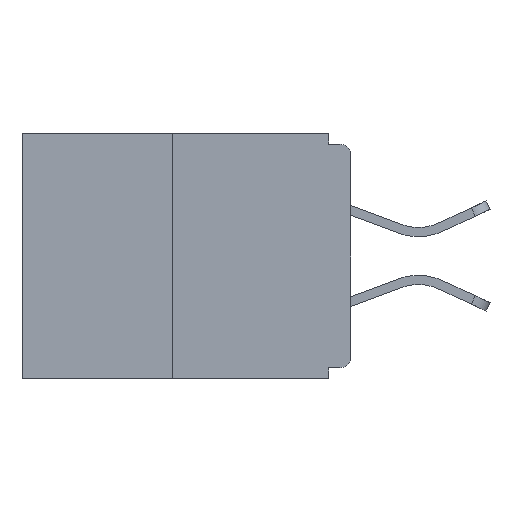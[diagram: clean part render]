
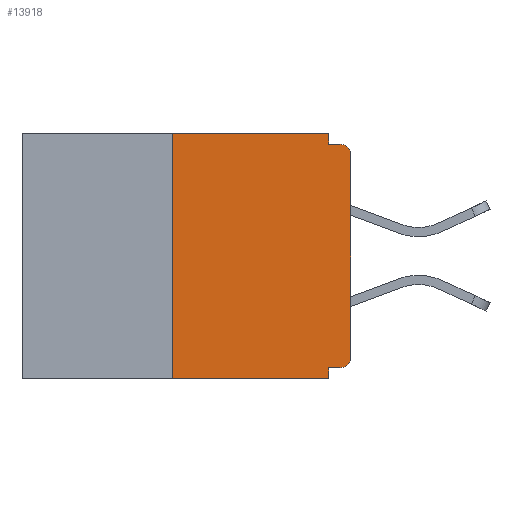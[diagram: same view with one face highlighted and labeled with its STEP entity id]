
A CAD part, left-side view. The second image highlights one B-rep face of the part: STEP entity #13918.
In plain terms, the highlighted planar face has unit normal (-1, 0, 0).
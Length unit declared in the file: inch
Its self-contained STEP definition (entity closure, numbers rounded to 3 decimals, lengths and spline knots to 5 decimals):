
#244 = DIRECTION ( 'NONE',  ( 0., 0., -1. ) ) ;
#1269 = ORIENTED_EDGE ( 'NONE', *, *, #27297, .T. ) ;
#1451 = VECTOR ( 'NONE', #10110, 39.37008 ) ;
#1606 = EDGE_CURVE ( 'NONE', #27535, #6457, #12747, .T. ) ;
#1632 = LINE ( 'NONE', #20170, #25090 ) ;
#3318 = EDGE_CURVE ( 'NONE', #17421, #14112, #13396, .T. ) ;
#3349 = DIRECTION ( 'NONE',  ( 0., 1., 0. ) ) ;
#3446 = FACE_OUTER_BOUND ( 'NONE', #28514, .T. ) ;
#3827 = DIRECTION ( 'NONE',  ( -1., 0., 0. ) ) ;
#4696 = CARTESIAN_POINT ( 'NONE',  ( 0., 0., -0.03 ) ) ;
#4707 = EDGE_CURVE ( 'NONE', #17421, #27535, #1632, .T. ) ;
#4799 = DIRECTION ( 'NONE',  ( 0., 0., 1. ) ) ;
#4879 = CARTESIAN_POINT ( 'NONE',  ( 0., 0.015, -0.015 ) ) ;
#5597 = ORIENTED_EDGE ( 'NONE', *, *, #26830, .F. ) ;
#5792 = DIRECTION ( 'NONE',  ( 0., -1., 0. ) ) ;
#6457 = VERTEX_POINT ( 'NONE', #23678 ) ;
#6660 = DIRECTION ( 'NONE',  ( 0., 0., -1. ) ) ;
#7023 = VECTOR ( 'NONE', #22921, 39.37008 ) ;
#7304 = ORIENTED_EDGE ( 'NONE', *, *, #18194, .T. ) ;
#7591 = LINE ( 'NONE', #8081, #26158 ) ;
#8001 = CARTESIAN_POINT ( 'NONE',  ( 0., 0.46, -0.343 ) ) ;
#8081 = CARTESIAN_POINT ( 'NONE',  ( 0., 0.46, 0. ) ) ;
#8383 = ORIENTED_EDGE ( 'NONE', *, *, #1606, .F. ) ;
#8634 = DIRECTION ( 'NONE',  ( 0., 0., -1. ) ) ;
#10096 = EDGE_CURVE ( 'NONE', #23647, #10309, #16117, .T. ) ;
#10110 = DIRECTION ( 'NONE',  ( 0., -1., 0. ) ) ;
#10309 = VERTEX_POINT ( 'NONE', #4879 ) ;
#10665 = LINE ( 'NONE', #24945, #21324 ) ;
#10746 = LINE ( 'NONE', #24054, #30804 ) ;
#11079 = CARTESIAN_POINT ( 'NONE',  ( 0., 0.031, -0.328 ) ) ;
#11236 = VERTEX_POINT ( 'NONE', #28906 ) ;
#11507 = DIRECTION ( 'NONE',  ( 1., 0., 0. ) ) ;
#12478 = CARTESIAN_POINT ( 'NONE',  ( 0., 0.015, -0.03 ) ) ;
#12747 = LINE ( 'NONE', #18558, #24883 ) ;
#13314 = ORIENTED_EDGE ( 'NONE', *, *, #10096, .F. ) ;
#13396 = CIRCLE ( 'NONE', #30760, 0.015 ) ;
#13464 = AXIS2_PLACEMENT_3D ( 'NONE', #12478, #17383, #244 ) ;
#13481 = EDGE_CURVE ( 'NONE', #25976, #24935, #7591, .T. ) ;
#13722 = CARTESIAN_POINT ( 'NONE',  ( 0., 0.46, 0. ) ) ;
#13731 = CARTESIAN_POINT ( 'NONE',  ( 0., 0.031, 0. ) ) ;
#13918 = ADVANCED_FACE ( 'NONE', ( #3446 ), #28317, .F. ) ;
#14112 = VERTEX_POINT ( 'NONE', #22604 ) ;
#15017 = ORIENTED_EDGE ( 'NONE', *, *, #4707, .F. ) ;
#16117 = LINE ( 'NONE', #22476, #7023 ) ;
#16212 = DIRECTION ( 'NONE',  ( 0., 0., -1. ) ) ;
#16394 = DIRECTION ( 'NONE',  ( 0., 0., -1. ) ) ;
#16592 = CARTESIAN_POINT ( 'NONE',  ( 0., 0.25, 0. ) ) ;
#17383 = DIRECTION ( 'NONE',  ( -1., 0., 0. ) ) ;
#17421 = VERTEX_POINT ( 'NONE', #30792 ) ;
#17628 = CIRCLE ( 'NONE', #13464, 0.015 ) ;
#18149 = LINE ( 'NONE', #13731, #29032 ) ;
#18194 = EDGE_CURVE ( 'NONE', #20850, #10309, #17628, .T. ) ;
#18321 = CARTESIAN_POINT ( 'NONE',  ( 0., 0.015, -0.313 ) ) ;
#18558 = CARTESIAN_POINT ( 'NONE',  ( 0., 0.031, -0.343 ) ) ;
#18849 = CARTESIAN_POINT ( 'NONE',  ( 0., 0.031, -0.015 ) ) ;
#18994 = ORIENTED_EDGE ( 'NONE', *, *, #3318, .T. ) ;
#19004 = EDGE_CURVE ( 'NONE', #11236, #25976, #10746, .T. ) ;
#20170 = CARTESIAN_POINT ( 'NONE',  ( 0., 0., -0.328 ) ) ;
#20850 = VERTEX_POINT ( 'NONE', #4696 ) ;
#20882 = CARTESIAN_POINT ( 'NONE',  ( 0., 0.031, 0. ) ) ;
#21324 = VECTOR ( 'NONE', #22397, 39.37008 ) ;
#22397 = DIRECTION ( 'NONE',  ( 0., 0., 1. ) ) ;
#22476 = CARTESIAN_POINT ( 'NONE',  ( 0., 0., -0.015 ) ) ;
#22604 = CARTESIAN_POINT ( 'NONE',  ( 0., 0., -0.313 ) ) ;
#22921 = DIRECTION ( 'NONE',  ( 0., -1., 0. ) ) ;
#23647 = VERTEX_POINT ( 'NONE', #18849 ) ;
#23678 = CARTESIAN_POINT ( 'NONE',  ( 0., 0.031, -0.343 ) ) ;
#23843 = EDGE_CURVE ( 'NONE', #14112, #20850, #10665, .T. ) ;
#24054 = CARTESIAN_POINT ( 'NONE',  ( 0., 0.25, 0. ) ) ;
#24883 = VECTOR ( 'NONE', #16212, 39.37008 ) ;
#24935 = VERTEX_POINT ( 'NONE', #20882 ) ;
#24945 = CARTESIAN_POINT ( 'NONE',  ( 0., 0., 0. ) ) ;
#25090 = VECTOR ( 'NONE', #3349, 39.37008 ) ;
#25240 = ORIENTED_EDGE ( 'NONE', *, *, #19004, .F. ) ;
#25298 = LINE ( 'NONE', #8001, #1451 ) ;
#25976 = VERTEX_POINT ( 'NONE', #16592 ) ;
#26158 = VECTOR ( 'NONE', #5792, 39.37008 ) ;
#26830 = EDGE_CURVE ( 'NONE', #24935, #23647, #18149, .T. ) ;
#26951 = AXIS2_PLACEMENT_3D ( 'NONE', #13722, #11507, #16394 ) ;
#27297 = EDGE_CURVE ( 'NONE', #11236, #6457, #25298, .T. ) ;
#27535 = VERTEX_POINT ( 'NONE', #11079 ) ;
#28317 = PLANE ( 'NONE',  #26951 ) ;
#28409 = ORIENTED_EDGE ( 'NONE', *, *, #23843, .T. ) ;
#28514 = EDGE_LOOP ( 'NONE', ( #30448, #25240, #1269, #8383, #15017, #18994, #28409, #7304, #13314, #5597 ) ) ;
#28906 = CARTESIAN_POINT ( 'NONE',  ( 0., 0.25, -0.343 ) ) ;
#29032 = VECTOR ( 'NONE', #6660, 39.37008 ) ;
#30448 = ORIENTED_EDGE ( 'NONE', *, *, #13481, .F. ) ;
#30760 = AXIS2_PLACEMENT_3D ( 'NONE', #18321, #3827, #8634 ) ;
#30792 = CARTESIAN_POINT ( 'NONE',  ( 0., 0.015, -0.328 ) ) ;
#30804 = VECTOR ( 'NONE', #4799, 39.37008 ) ;
